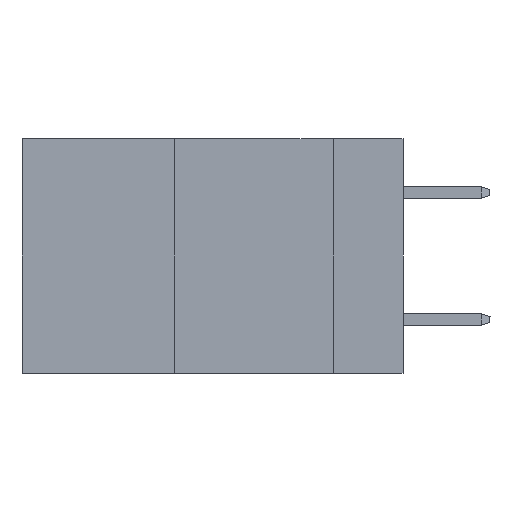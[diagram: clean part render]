
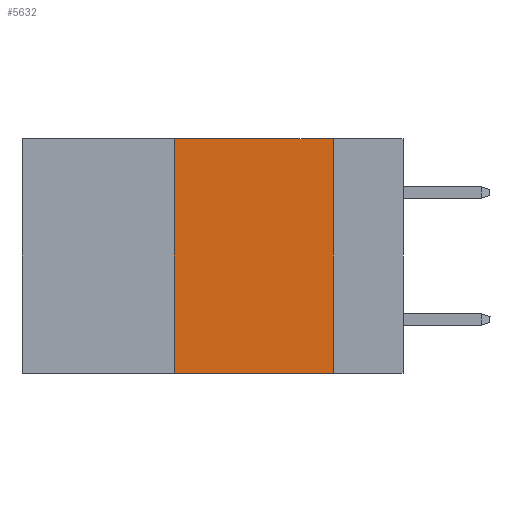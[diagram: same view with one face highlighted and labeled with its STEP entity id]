
A CAD part, left-side view. The second image highlights one B-rep face of the part: STEP entity #5632.
In plain terms, the highlighted planar face has unit normal (-1, 0, 0).
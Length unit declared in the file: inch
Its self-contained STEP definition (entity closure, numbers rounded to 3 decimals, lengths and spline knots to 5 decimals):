
#4598 = EDGE_LOOP ( 'NONE', ( #27402, #33201, #6504, #24294 ) ) ;
#4934 = EDGE_CURVE ( 'NONE', #36587, #15366, #34748, .T. ) ;
#5632 = ADVANCED_FACE ( 'NONE', ( #20129 ), #28821, .F. ) ;
#6504 = ORIENTED_EDGE ( 'NONE', *, *, #15849, .F. ) ;
#7161 = VERTEX_POINT ( 'NONE', #16975 ) ;
#7210 = CARTESIAN_POINT ( 'NONE',  ( 0., 0.11, -0.37 ) ) ;
#8013 = VECTOR ( 'NONE', #15085, 39.37008 ) ;
#8591 = CARTESIAN_POINT ( 'NONE',  ( 0., 0.11, 0. ) ) ;
#9685 = VECTOR ( 'NONE', #14430, 39.37008 ) ;
#10495 = VERTEX_POINT ( 'NONE', #33662 ) ;
#13406 = CARTESIAN_POINT ( 'NONE',  ( 0., 0.6, 0. ) ) ;
#14430 = DIRECTION ( 'NONE',  ( 0., -1., 0. ) ) ;
#15085 = DIRECTION ( 'NONE',  ( 0., 0., 1. ) ) ;
#15103 = DIRECTION ( 'NONE',  ( 0., 0., -1. ) ) ;
#15366 = VERTEX_POINT ( 'NONE', #7210 ) ;
#15849 = EDGE_CURVE ( 'NONE', #10495, #7161, #34103, .T. ) ;
#16975 = CARTESIAN_POINT ( 'NONE',  ( 0., 0.36, 0. ) ) ;
#20129 = FACE_OUTER_BOUND ( 'NONE', #4598, .T. ) ;
#20605 = VECTOR ( 'NONE', #15103, 39.37008 ) ;
#22861 = CARTESIAN_POINT ( 'NONE',  ( 0., 0.6, 0. ) ) ;
#23297 = DIRECTION ( 'NONE',  ( 0., -1., 0. ) ) ;
#24294 = ORIENTED_EDGE ( 'NONE', *, *, #38499, .T. ) ;
#25221 = CARTESIAN_POINT ( 'NONE',  ( 0., 0.11, 0. ) ) ;
#25637 = DIRECTION ( 'NONE',  ( 1., 0., 0. ) ) ;
#27402 = ORIENTED_EDGE ( 'NONE', *, *, #4934, .F. ) ;
#28580 = VECTOR ( 'NONE', #23297, 39.37008 ) ;
#28821 = PLANE ( 'NONE',  #36747 ) ;
#30871 = CARTESIAN_POINT ( 'NONE',  ( 0., 0.6, -0.37 ) ) ;
#32910 = EDGE_CURVE ( 'NONE', #7161, #36587, #36414, .T. ) ;
#33201 = ORIENTED_EDGE ( 'NONE', *, *, #32910, .F. ) ;
#33662 = CARTESIAN_POINT ( 'NONE',  ( 0., 0.36, -0.37 ) ) ;
#34103 = LINE ( 'NONE', #34312, #8013 ) ;
#34312 = CARTESIAN_POINT ( 'NONE',  ( 0., 0.36, 0. ) ) ;
#34748 = LINE ( 'NONE', #25221, #20605 ) ;
#35376 = DIRECTION ( 'NONE',  ( 0., 0., -1. ) ) ;
#36414 = LINE ( 'NONE', #13406, #28580 ) ;
#36587 = VERTEX_POINT ( 'NONE', #8591 ) ;
#36747 = AXIS2_PLACEMENT_3D ( 'NONE', #22861, #25637, #35376 ) ;
#38499 = EDGE_CURVE ( 'NONE', #10495, #15366, #40813, .T. ) ;
#40813 = LINE ( 'NONE', #30871, #9685 ) ;
